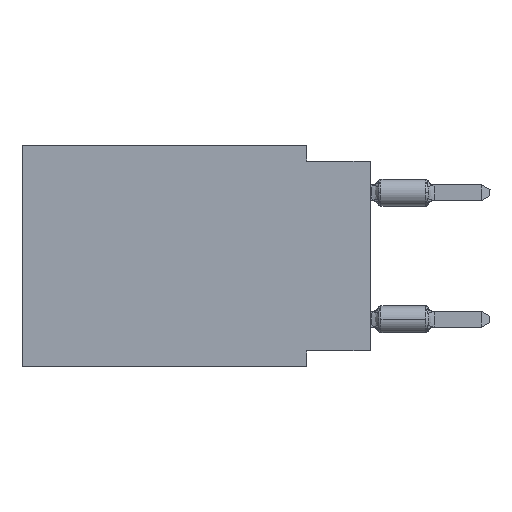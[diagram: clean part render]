
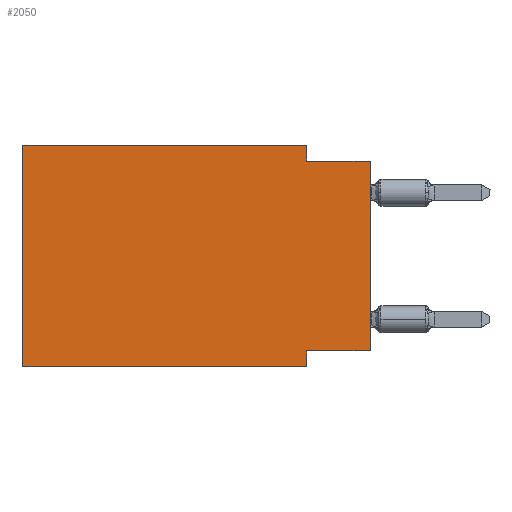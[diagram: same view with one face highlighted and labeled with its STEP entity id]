
A CAD part, left-side view. The second image highlights one B-rep face of the part: STEP entity #2050.
In plain terms, the highlighted planar face has unit normal (-1, 0, 0).
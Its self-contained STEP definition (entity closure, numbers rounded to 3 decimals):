
#54 = LINE ( 'NONE', #31821, #28445 ) ;
#245 = EDGE_CURVE ( 'NONE', #16714, #18580, #37038, .T. ) ;
#1137 = EDGE_CURVE ( 'NONE', #6545, #18167, #10850, .T. ) ;
#1656 = PLANE ( 'NONE',  #12023 ) ;
#1872 = DIRECTION ( 'NONE',  ( 0., 0., 1. ) ) ;
#2050 = ADVANCED_FACE ( 'NONE', ( #35895 ), #1656, .F. ) ;
#2280 = EDGE_CURVE ( 'NONE', #21040, #18167, #6385, .T. ) ;
#2751 = ORIENTED_EDGE ( 'NONE', *, *, #28929, .F. ) ;
#2935 = VECTOR ( 'NONE', #15696, 1000. ) ;
#3262 = ORIENTED_EDGE ( 'NONE', *, *, #1137, .T. ) ;
#3266 = ORIENTED_EDGE ( 'NONE', *, *, #2280, .F. ) ;
#3321 = CARTESIAN_POINT ( 'NONE',  ( 0., 0., -0.635 ) ) ;
#4099 = CARTESIAN_POINT ( 'NONE',  ( 0., 0., -8.255 ) ) ;
#4518 = DIRECTION ( 'NONE',  ( 0., -1., 0. ) ) ;
#4585 = ORIENTED_EDGE ( 'NONE', *, *, #21999, .F. ) ;
#5382 = CARTESIAN_POINT ( 'NONE',  ( 0., 2.54, 0. ) ) ;
#6385 = LINE ( 'NONE', #3321, #12625 ) ;
#6545 = VERTEX_POINT ( 'NONE', #9752 ) ;
#6740 = VERTEX_POINT ( 'NONE', #11416 ) ;
#7151 = LINE ( 'NONE', #4099, #2935 ) ;
#7269 = DIRECTION ( 'NONE',  ( 0., 0., 1. ) ) ;
#7369 = DIRECTION ( 'NONE',  ( 1., 0., 0. ) ) ;
#7483 = VECTOR ( 'NONE', #7269, 1000. ) ;
#8792 = CARTESIAN_POINT ( 'NONE',  ( 0., 2.54, -8.89 ) ) ;
#9088 = CARTESIAN_POINT ( 'NONE',  ( 0., 2.54, 0. ) ) ;
#9720 = VECTOR ( 'NONE', #4518, 1000. ) ;
#9752 = CARTESIAN_POINT ( 'NONE',  ( 0., 0., -8.255 ) ) ;
#10101 = CARTESIAN_POINT ( 'NONE',  ( 0., 2.54, -8.89 ) ) ;
#10152 = CARTESIAN_POINT ( 'NONE',  ( 0., 0., -0.635 ) ) ;
#10381 = ORIENTED_EDGE ( 'NONE', *, *, #24596, .F. ) ;
#10850 = LINE ( 'NONE', #33318, #7483 ) ;
#11416 = CARTESIAN_POINT ( 'NONE',  ( 0., 2.54, -8.255 ) ) ;
#12023 = AXIS2_PLACEMENT_3D ( 'NONE', #18781, #7369, #33232 ) ;
#12625 = VECTOR ( 'NONE', #14913, 1000. ) ;
#13058 = ORIENTED_EDGE ( 'NONE', *, *, #245, .T. ) ;
#13190 = CARTESIAN_POINT ( 'NONE',  ( 0., 13.97, 0. ) ) ;
#13279 = CARTESIAN_POINT ( 'NONE',  ( 0., 13.97, 0. ) ) ;
#13682 = VERTEX_POINT ( 'NONE', #9088 ) ;
#14913 = DIRECTION ( 'NONE',  ( 0., -1., 0. ) ) ;
#15696 = DIRECTION ( 'NONE',  ( 0., 1., 0. ) ) ;
#16714 = VERTEX_POINT ( 'NONE', #25390 ) ;
#17067 = VECTOR ( 'NONE', #1872, 1000. ) ;
#17910 = CARTESIAN_POINT ( 'NONE',  ( 0., 2.54, -0.635 ) ) ;
#18167 = VERTEX_POINT ( 'NONE', #10152 ) ;
#18210 = VERTEX_POINT ( 'NONE', #13190 ) ;
#18580 = VERTEX_POINT ( 'NONE', #10101 ) ;
#18781 = CARTESIAN_POINT ( 'NONE',  ( 0., 13.97, 0. ) ) ;
#20963 = LINE ( 'NONE', #8792, #33123 ) ;
#21040 = VERTEX_POINT ( 'NONE', #17910 ) ;
#21562 = EDGE_CURVE ( 'NONE', #16714, #18210, #36311, .T. ) ;
#21999 = EDGE_CURVE ( 'NONE', #13682, #21040, #34296, .T. ) ;
#24596 = EDGE_CURVE ( 'NONE', #6545, #6740, #7151, .T. ) ;
#25390 = CARTESIAN_POINT ( 'NONE',  ( 0., 13.97, -8.89 ) ) ;
#25546 = DIRECTION ( 'NONE',  ( 0., 0., -1. ) ) ;
#26291 = DIRECTION ( 'NONE',  ( 0., 0., -1. ) ) ;
#26789 = VECTOR ( 'NONE', #25546, 1000. ) ;
#27827 = EDGE_LOOP ( 'NONE', ( #3262, #3266, #4585, #36489, #32451, #13058, #2751, #10381 ) ) ;
#28445 = VECTOR ( 'NONE', #29345, 1000. ) ;
#28929 = EDGE_CURVE ( 'NONE', #6740, #18580, #20963, .T. ) ;
#29345 = DIRECTION ( 'NONE',  ( 0., -1., 0. ) ) ;
#30579 = CARTESIAN_POINT ( 'NONE',  ( 0., 13.97, -8.89 ) ) ;
#31821 = CARTESIAN_POINT ( 'NONE',  ( 0., 13.97, 0. ) ) ;
#32259 = EDGE_CURVE ( 'NONE', #18210, #13682, #54, .T. ) ;
#32451 = ORIENTED_EDGE ( 'NONE', *, *, #21562, .F. ) ;
#33123 = VECTOR ( 'NONE', #26291, 1000. ) ;
#33232 = DIRECTION ( 'NONE',  ( 0., 0., -1. ) ) ;
#33318 = CARTESIAN_POINT ( 'NONE',  ( 0., 0., 0. ) ) ;
#34296 = LINE ( 'NONE', #5382, #26789 ) ;
#35895 = FACE_OUTER_BOUND ( 'NONE', #27827, .T. ) ;
#36311 = LINE ( 'NONE', #13279, #17067 ) ;
#36489 = ORIENTED_EDGE ( 'NONE', *, *, #32259, .F. ) ;
#37038 = LINE ( 'NONE', #30579, #9720 ) ;
